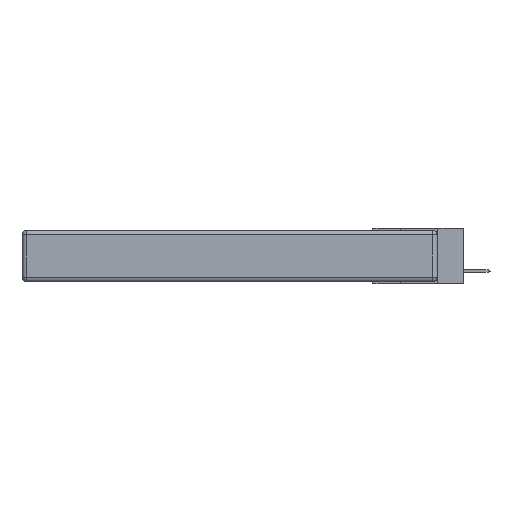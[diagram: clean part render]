
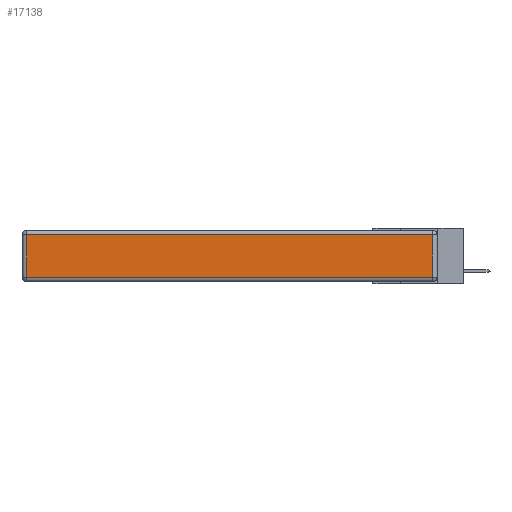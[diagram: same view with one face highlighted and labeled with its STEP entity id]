
A CAD part, left-side view. The second image highlights one B-rep face of the part: STEP entity #17138.
In plain terms, the highlighted planar face has unit normal (-1, 0, 0).
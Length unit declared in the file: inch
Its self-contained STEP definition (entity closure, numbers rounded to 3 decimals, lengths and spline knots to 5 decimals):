
#1217 = EDGE_CURVE ( 'NONE', #19683, #11457, #3789, .T. ) ;
#1625 = CARTESIAN_POINT ( 'NONE',  ( 0., 0., -0.343 ) ) ;
#1714 = FACE_OUTER_BOUND ( 'NONE', #18175, .T. ) ;
#2898 = VECTOR ( 'NONE', #12865, 39.37008 ) ;
#3571 = DIRECTION ( 'NONE',  ( 0., 0., 1. ) ) ;
#3789 = LINE ( 'NONE', #15377, #2898 ) ;
#4394 = CARTESIAN_POINT ( 'NONE',  ( 0., 2.72, -0.03 ) ) ;
#4704 = CARTESIAN_POINT ( 'NONE',  ( 0., 2.75, -0.03 ) ) ;
#5617 = LINE ( 'NONE', #18679, #16536 ) ;
#5969 = EDGE_CURVE ( 'NONE', #15448, #19683, #21092, .T. ) ;
#8337 = ORIENTED_EDGE ( 'NONE', *, *, #15728, .T. ) ;
#8765 = VERTEX_POINT ( 'NONE', #9639 ) ;
#9022 = DIRECTION ( 'NONE',  ( 0., 0., 1. ) ) ;
#9639 = CARTESIAN_POINT ( 'NONE',  ( 0., 0.03, -0.313 ) ) ;
#9776 = ORIENTED_EDGE ( 'NONE', *, *, #5969, .T. ) ;
#11191 = PLANE ( 'NONE',  #23783 ) ;
#11417 = CARTESIAN_POINT ( 'NONE',  ( 0., 2.72, -0.313 ) ) ;
#11457 = VERTEX_POINT ( 'NONE', #11417 ) ;
#12277 = CARTESIAN_POINT ( 'NONE',  ( 0., 0.03, -0.03 ) ) ;
#12865 = DIRECTION ( 'NONE',  ( 0., 0., -1. ) ) ;
#13378 = DIRECTION ( 'NONE',  ( 0., -1., 0. ) ) ;
#13566 = VECTOR ( 'NONE', #18291, 39.37008 ) ;
#13759 = ORIENTED_EDGE ( 'NONE', *, *, #23085, .T. ) ;
#15179 = DIRECTION ( 'NONE',  ( -1., 0., 0. ) ) ;
#15292 = VECTOR ( 'NONE', #13378, 39.37008 ) ;
#15341 = CARTESIAN_POINT ( 'NONE',  ( 0., 0., -0.313 ) ) ;
#15377 = CARTESIAN_POINT ( 'NONE',  ( 0., 2.72, -0.343 ) ) ;
#15448 = VERTEX_POINT ( 'NONE', #12277 ) ;
#15728 = EDGE_CURVE ( 'NONE', #8765, #15448, #5617, .T. ) ;
#16509 = LINE ( 'NONE', #15341, #15292 ) ;
#16536 = VECTOR ( 'NONE', #9022, 39.37008 ) ;
#17138 = ADVANCED_FACE ( 'NONE', ( #1714 ), #11191, .T. ) ;
#18175 = EDGE_LOOP ( 'NONE', ( #13759, #8337, #9776, #19900 ) ) ;
#18291 = DIRECTION ( 'NONE',  ( 0., 1., 0. ) ) ;
#18679 = CARTESIAN_POINT ( 'NONE',  ( 0., 0.03, -0.343 ) ) ;
#19683 = VERTEX_POINT ( 'NONE', #4394 ) ;
#19900 = ORIENTED_EDGE ( 'NONE', *, *, #1217, .T. ) ;
#21092 = LINE ( 'NONE', #4704, #13566 ) ;
#23085 = EDGE_CURVE ( 'NONE', #11457, #8765, #16509, .T. ) ;
#23783 = AXIS2_PLACEMENT_3D ( 'NONE', #1625, #15179, #3571 ) ;
